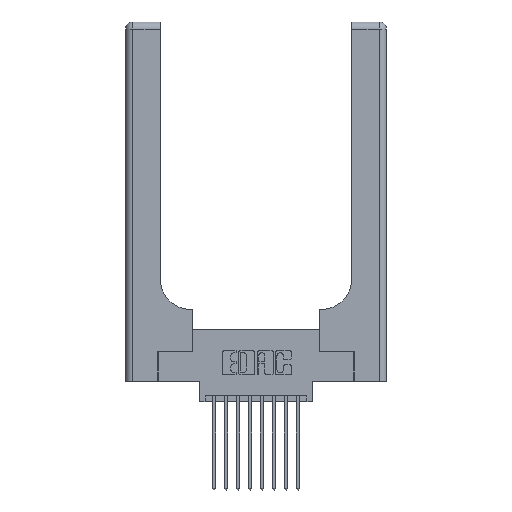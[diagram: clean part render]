
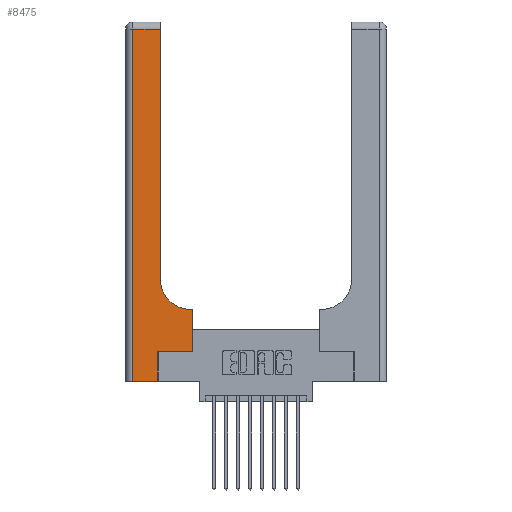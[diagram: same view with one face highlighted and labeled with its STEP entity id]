
A CAD part, top view. The second image highlights one B-rep face of the part: STEP entity #8475.
In plain terms, the highlighted planar face has unit normal (0, 0, 1).
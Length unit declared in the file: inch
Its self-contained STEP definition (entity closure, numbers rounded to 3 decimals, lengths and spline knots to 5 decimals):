
#15 = DIRECTION ( 'NONE',  ( 0., 1., 0. ) ) ;
#46 = LINE ( 'NONE', #3501, #9791 ) ;
#597 = LINE ( 'NONE', #9898, #13522 ) ;
#894 = LINE ( 'NONE', #6025, #3835 ) ;
#931 = EDGE_CURVE ( 'NONE', #15951, #14825, #11582, .T. ) ;
#1789 = ORIENTED_EDGE ( 'NONE', *, *, #931, .T. ) ;
#1982 = DIRECTION ( 'NONE',  ( 0., 1., 0. ) ) ;
#2554 = EDGE_LOOP ( 'NONE', ( #14297, #1789, #8932, #9337, #12937, #3359, #7187, #4563, #8344 ) ) ;
#2772 = CARTESIAN_POINT ( 'NONE',  ( 0.06, 2.94, 0.37 ) ) ;
#3320 = DIRECTION ( 'NONE',  ( 0., -1., 0. ) ) ;
#3349 = VECTOR ( 'NONE', #10469, 39.37008 ) ;
#3359 = ORIENTED_EDGE ( 'NONE', *, *, #13746, .T. ) ;
#3501 = CARTESIAN_POINT ( 'NONE',  ( 0., 0., 0.37 ) ) ;
#3751 = LINE ( 'NONE', #9229, #3349 ) ;
#3835 = VECTOR ( 'NONE', #8535, 39.37008 ) ;
#3951 = CARTESIAN_POINT ( 'NONE',  ( 0.06, 0., 0.37 ) ) ;
#4326 = EDGE_CURVE ( 'NONE', #6404, #13163, #46, .T. ) ;
#4443 = CARTESIAN_POINT ( 'NONE',  ( 0., 2.94, 0.37 ) ) ;
#4490 = CARTESIAN_POINT ( 'NONE',  ( 0.5585, 0.6, 0.37 ) ) ;
#4563 = ORIENTED_EDGE ( 'NONE', *, *, #9212, .T. ) ;
#4689 = DIRECTION ( 'NONE',  ( 0., 0., -1. ) ) ;
#5238 = CIRCLE ( 'NONE', #15372, 0.25 ) ;
#5950 = CARTESIAN_POINT ( 'NONE',  ( 0., 3., 0.37 ) ) ;
#5988 = VECTOR ( 'NONE', #15, 39.37008 ) ;
#6025 = CARTESIAN_POINT ( 'NONE',  ( 0.269, 0.25, 0.37 ) ) ;
#6399 = CARTESIAN_POINT ( 'NONE',  ( 0.2915, 3., 0.37 ) ) ;
#6404 = VERTEX_POINT ( 'NONE', #3951 ) ;
#6473 = DIRECTION ( 'NONE',  ( -1., 0., 0. ) ) ;
#6561 = VERTEX_POINT ( 'NONE', #7725 ) ;
#7046 = EDGE_CURVE ( 'NONE', #10390, #15951, #9733, .T. ) ;
#7181 = CARTESIAN_POINT ( 'NONE',  ( 0.2915, 0.85, 0.37 ) ) ;
#7187 = ORIENTED_EDGE ( 'NONE', *, *, #9477, .T. ) ;
#7232 = DIRECTION ( 'NONE',  ( 0., 0., -1. ) ) ;
#7520 = VERTEX_POINT ( 'NONE', #12316 ) ;
#7725 = CARTESIAN_POINT ( 'NONE',  ( 0.5585, 0.25, 0.37 ) ) ;
#8133 = LINE ( 'NONE', #12021, #11058 ) ;
#8344 = ORIENTED_EDGE ( 'NONE', *, *, #14208, .T. ) ;
#8475 = ADVANCED_FACE ( 'NONE', ( #12213 ), #13338, .F. ) ;
#8535 = DIRECTION ( 'NONE',  ( 1., 0., 0. ) ) ;
#8722 = CARTESIAN_POINT ( 'NONE',  ( 0.2915, 2.94, 0.37 ) ) ;
#8932 = ORIENTED_EDGE ( 'NONE', *, *, #11447, .T. ) ;
#9008 = VERTEX_POINT ( 'NONE', #10748 ) ;
#9087 = LINE ( 'NONE', #13305, #11946 ) ;
#9212 = EDGE_CURVE ( 'NONE', #14393, #9008, #597, .T. ) ;
#9229 = CARTESIAN_POINT ( 'NONE',  ( 0.5585, 0.25, 0.37 ) ) ;
#9337 = ORIENTED_EDGE ( 'NONE', *, *, #4326, .T. ) ;
#9463 = CARTESIAN_POINT ( 'NONE',  ( 0.269, 0., 0.37 ) ) ;
#9477 = EDGE_CURVE ( 'NONE', #6561, #14393, #3751, .T. ) ;
#9733 = LINE ( 'NONE', #6399, #5988 ) ;
#9791 = VECTOR ( 'NONE', #9841, 39.37008 ) ;
#9837 = DIRECTION ( 'NONE',  ( -1., 0., 0. ) ) ;
#9841 = DIRECTION ( 'NONE',  ( 1., 0., 0. ) ) ;
#9898 = CARTESIAN_POINT ( 'NONE',  ( 0.2915, 0.6, 0.37 ) ) ;
#10340 = EDGE_CURVE ( 'NONE', #13163, #7520, #8133, .T. ) ;
#10390 = VERTEX_POINT ( 'NONE', #7181 ) ;
#10469 = DIRECTION ( 'NONE',  ( 0., 1., 0. ) ) ;
#10748 = CARTESIAN_POINT ( 'NONE',  ( 0.5415, 0.6, 0.37 ) ) ;
#11058 = VECTOR ( 'NONE', #1982, 39.37008 ) ;
#11447 = EDGE_CURVE ( 'NONE', #14825, #6404, #9087, .T. ) ;
#11582 = LINE ( 'NONE', #4443, #14857 ) ;
#11946 = VECTOR ( 'NONE', #3320, 39.37008 ) ;
#12021 = CARTESIAN_POINT ( 'NONE',  ( 0.269, 0., 0.37 ) ) ;
#12181 = CARTESIAN_POINT ( 'NONE',  ( 0.5415, 0.85, 0.37 ) ) ;
#12213 = FACE_OUTER_BOUND ( 'NONE', #2554, .T. ) ;
#12316 = CARTESIAN_POINT ( 'NONE',  ( 0.269, 0.25, 0.37 ) ) ;
#12937 = ORIENTED_EDGE ( 'NONE', *, *, #10340, .T. ) ;
#13163 = VERTEX_POINT ( 'NONE', #9463 ) ;
#13216 = AXIS2_PLACEMENT_3D ( 'NONE', #5950, #7232, #15831 ) ;
#13305 = CARTESIAN_POINT ( 'NONE',  ( 0.06, 3., 0.37 ) ) ;
#13338 = PLANE ( 'NONE',  #13216 ) ;
#13392 = DIRECTION ( 'NONE',  ( 1., 0., 0. ) ) ;
#13522 = VECTOR ( 'NONE', #9837, 39.37008 ) ;
#13746 = EDGE_CURVE ( 'NONE', #7520, #6561, #894, .T. ) ;
#14208 = EDGE_CURVE ( 'NONE', #9008, #10390, #5238, .T. ) ;
#14297 = ORIENTED_EDGE ( 'NONE', *, *, #7046, .T. ) ;
#14393 = VERTEX_POINT ( 'NONE', #4490 ) ;
#14825 = VERTEX_POINT ( 'NONE', #2772 ) ;
#14857 = VECTOR ( 'NONE', #6473, 39.37008 ) ;
#15372 = AXIS2_PLACEMENT_3D ( 'NONE', #12181, #4689, #13392 ) ;
#15831 = DIRECTION ( 'NONE',  ( -1., 0., 0. ) ) ;
#15951 = VERTEX_POINT ( 'NONE', #8722 ) ;
